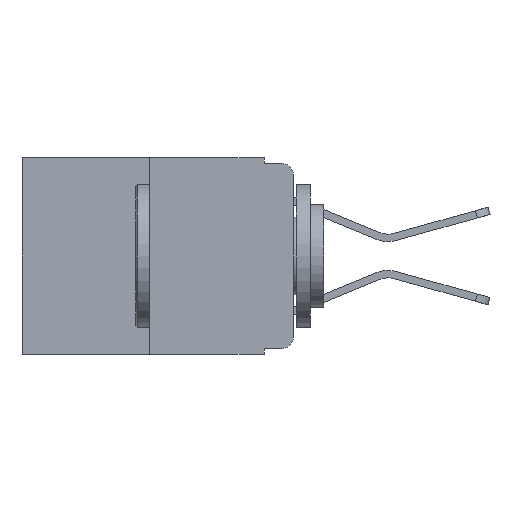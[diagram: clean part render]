
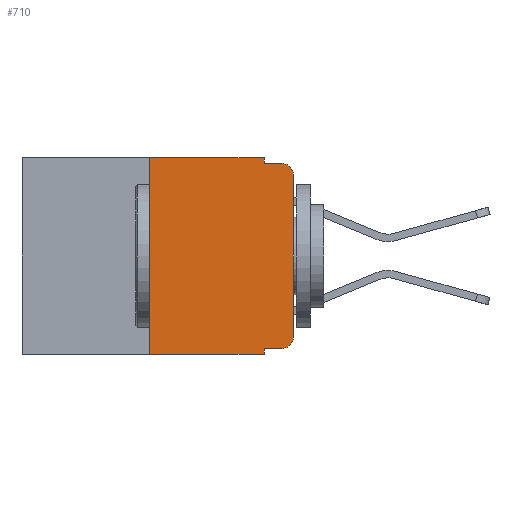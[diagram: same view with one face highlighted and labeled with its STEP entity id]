
A CAD part, left-side view. The second image highlights one B-rep face of the part: STEP entity #710.
In plain terms, the highlighted planar face has unit normal (-1, 0, 0).
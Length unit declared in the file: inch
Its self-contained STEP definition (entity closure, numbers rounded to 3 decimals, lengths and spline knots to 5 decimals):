
#163 = VECTOR ( 'NONE', #9078, 39.37008 ) ;
#193 = CARTESIAN_POINT ( 'NONE',  ( 0., 0.051, -0.01 ) ) ;
#432 = CARTESIAN_POINT ( 'NONE',  ( 0., 0.473, 0. ) ) ;
#710 = ADVANCED_FACE ( 'NONE', ( #9310 ), #10971, .F. ) ;
#941 = CARTESIAN_POINT ( 'NONE',  ( 0., 0.02, -0.333 ) ) ;
#1249 = LINE ( 'NONE', #1562, #11010 ) ;
#1462 = LINE ( 'NONE', #193, #10902 ) ;
#1536 = VECTOR ( 'NONE', #7771, 39.37008 ) ;
#1562 = CARTESIAN_POINT ( 'NONE',  ( 0., 0.051, 0. ) ) ;
#2208 = DIRECTION ( 'NONE',  ( -1., 0., 0. ) ) ;
#2275 = CARTESIAN_POINT ( 'NONE',  ( 0., 0.25, 0. ) ) ;
#2335 = CARTESIAN_POINT ( 'NONE',  ( 0., 0., -0.313 ) ) ;
#2510 = DIRECTION ( 'NONE',  ( 0., -1., 0. ) ) ;
#2600 = EDGE_CURVE ( 'NONE', #5800, #8786, #3148, .T. ) ;
#2698 = ORIENTED_EDGE ( 'NONE', *, *, #5265, .F. ) ;
#2856 = CARTESIAN_POINT ( 'NONE',  ( 0., 0.473, 0. ) ) ;
#2914 = CARTESIAN_POINT ( 'NONE',  ( 0., 0.051, 0. ) ) ;
#3003 = ORIENTED_EDGE ( 'NONE', *, *, #2600, .T. ) ;
#3148 = LINE ( 'NONE', #11069, #163 ) ;
#3216 = DIRECTION ( 'NONE',  ( -1., 0., 0. ) ) ;
#3222 = DIRECTION ( 'NONE',  ( 0., -1., 0. ) ) ;
#3430 = VECTOR ( 'NONE', #6264, 39.37008 ) ;
#3479 = CARTESIAN_POINT ( 'NONE',  ( 0., 0.051, -0.333 ) ) ;
#3718 = CARTESIAN_POINT ( 'NONE',  ( 0., 0.051, 0. ) ) ;
#3733 = CARTESIAN_POINT ( 'NONE',  ( 0., 0.25, -0.343 ) ) ;
#3767 = CARTESIAN_POINT ( 'NONE',  ( 0., 0.051, -0.01 ) ) ;
#4008 = EDGE_CURVE ( 'NONE', #5800, #4242, #4637, .T. ) ;
#4044 = CARTESIAN_POINT ( 'NONE',  ( 0., 0.02, -0.01 ) ) ;
#4054 = CARTESIAN_POINT ( 'NONE',  ( 0., 0., -0.03 ) ) ;
#4066 = CARTESIAN_POINT ( 'NONE',  ( 0., 0.051, -0.333 ) ) ;
#4074 = ORIENTED_EDGE ( 'NONE', *, *, #5075, .T. ) ;
#4115 = DIRECTION ( 'NONE',  ( 0., -1., 0. ) ) ;
#4143 = LINE ( 'NONE', #7651, #1536 ) ;
#4242 = VERTEX_POINT ( 'NONE', #2275 ) ;
#4418 = VERTEX_POINT ( 'NONE', #4044 ) ;
#4441 = VECTOR ( 'NONE', #11326, 39.37008 ) ;
#4610 = LINE ( 'NONE', #432, #11670 ) ;
#4637 = LINE ( 'NONE', #9195, #3430 ) ;
#4773 = CARTESIAN_POINT ( 'NONE',  ( 0., 0.051, -0.343 ) ) ;
#4924 = VERTEX_POINT ( 'NONE', #3767 ) ;
#4936 = VERTEX_POINT ( 'NONE', #4066 ) ;
#5075 = EDGE_CURVE ( 'NONE', #12012, #6615, #4143, .T. ) ;
#5265 = EDGE_CURVE ( 'NONE', #4242, #6402, #4610, .T. ) ;
#5486 = EDGE_LOOP ( 'NONE', ( #4074, #9021, #9306, #7163, #2698, #10190, #3003, #10468, #5860, #8597 ) ) ;
#5800 = VERTEX_POINT ( 'NONE', #3733 ) ;
#5860 = ORIENTED_EDGE ( 'NONE', *, *, #8612, .T. ) ;
#5914 = EDGE_CURVE ( 'NONE', #6402, #4924, #6918, .T. ) ;
#6145 = VECTOR ( 'NONE', #2510, 39.37008 ) ;
#6264 = DIRECTION ( 'NONE',  ( 0., 0., 1. ) ) ;
#6394 = AXIS2_PLACEMENT_3D ( 'NONE', #7884, #2208, #8816 ) ;
#6402 = VERTEX_POINT ( 'NONE', #3718 ) ;
#6435 = LINE ( 'NONE', #3479, #6145 ) ;
#6615 = VERTEX_POINT ( 'NONE', #4054 ) ;
#6918 = LINE ( 'NONE', #2914, #4441 ) ;
#7156 = AXIS2_PLACEMENT_3D ( 'NONE', #8809, #3216, #9743 ) ;
#7163 = ORIENTED_EDGE ( 'NONE', *, *, #5914, .F. ) ;
#7188 = VERTEX_POINT ( 'NONE', #941 ) ;
#7500 = DIRECTION ( 'NONE',  ( 0., 0., -1. ) ) ;
#7501 = DIRECTION ( 'NONE',  ( 1., 0., 0. ) ) ;
#7651 = CARTESIAN_POINT ( 'NONE',  ( 0., 0., 0. ) ) ;
#7771 = DIRECTION ( 'NONE',  ( 0., 0., 1. ) ) ;
#7884 = CARTESIAN_POINT ( 'NONE',  ( 0., 0.02, -0.313 ) ) ;
#8221 = DIRECTION ( 'NONE',  ( 0., 0., -1. ) ) ;
#8393 = EDGE_CURVE ( 'NONE', #4924, #4418, #1462, .T. ) ;
#8597 = ORIENTED_EDGE ( 'NONE', *, *, #11924, .T. ) ;
#8612 = EDGE_CURVE ( 'NONE', #4936, #7188, #6435, .T. ) ;
#8786 = VERTEX_POINT ( 'NONE', #4773 ) ;
#8809 = CARTESIAN_POINT ( 'NONE',  ( 0., 0.02, -0.03 ) ) ;
#8816 = DIRECTION ( 'NONE',  ( 0., 0., -1. ) ) ;
#9021 = ORIENTED_EDGE ( 'NONE', *, *, #10236, .T. ) ;
#9078 = DIRECTION ( 'NONE',  ( 0., -1., 0. ) ) ;
#9085 = AXIS2_PLACEMENT_3D ( 'NONE', #2856, #7501, #7500 ) ;
#9195 = CARTESIAN_POINT ( 'NONE',  ( 0., 0.25, 0. ) ) ;
#9306 = ORIENTED_EDGE ( 'NONE', *, *, #8393, .F. ) ;
#9310 = FACE_OUTER_BOUND ( 'NONE', #5486, .T. ) ;
#9743 = DIRECTION ( 'NONE',  ( 0., 0., -1. ) ) ;
#10190 = ORIENTED_EDGE ( 'NONE', *, *, #4008, .F. ) ;
#10236 = EDGE_CURVE ( 'NONE', #6615, #4418, #11437, .T. ) ;
#10467 = EDGE_CURVE ( 'NONE', #4936, #8786, #1249, .T. ) ;
#10468 = ORIENTED_EDGE ( 'NONE', *, *, #10467, .F. ) ;
#10902 = VECTOR ( 'NONE', #3222, 39.37008 ) ;
#10971 = PLANE ( 'NONE',  #9085 ) ;
#11010 = VECTOR ( 'NONE', #8221, 39.37008 ) ;
#11069 = CARTESIAN_POINT ( 'NONE',  ( 0., 0.473, -0.343 ) ) ;
#11326 = DIRECTION ( 'NONE',  ( 0., 0., -1. ) ) ;
#11437 = CIRCLE ( 'NONE', #7156, 0.02 ) ;
#11670 = VECTOR ( 'NONE', #4115, 39.37008 ) ;
#11678 = CIRCLE ( 'NONE', #6394, 0.02 ) ;
#11924 = EDGE_CURVE ( 'NONE', #7188, #12012, #11678, .T. ) ;
#12012 = VERTEX_POINT ( 'NONE', #2335 ) ;
